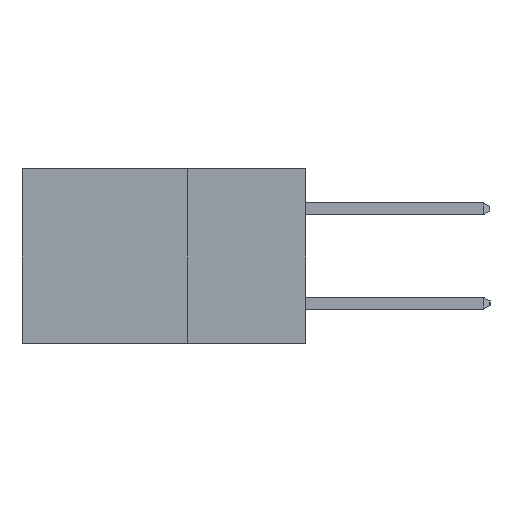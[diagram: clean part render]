
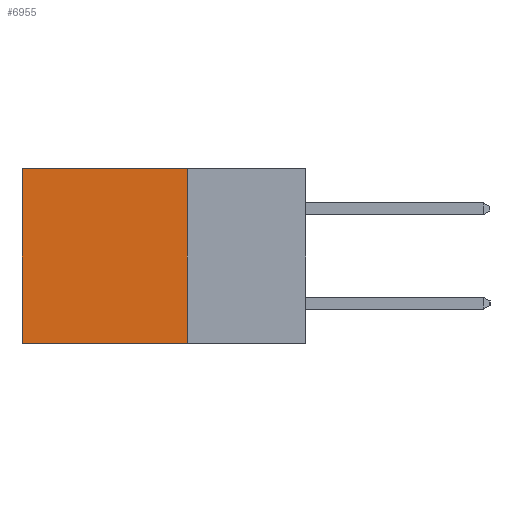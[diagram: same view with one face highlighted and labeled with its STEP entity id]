
A CAD part, left-side view. The second image highlights one B-rep face of the part: STEP entity #6955.
In plain terms, the highlighted planar face has unit normal (-1, 0, 0).
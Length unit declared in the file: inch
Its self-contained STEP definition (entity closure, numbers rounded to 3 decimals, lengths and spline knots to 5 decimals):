
#86 = DIRECTION ( 'NONE',  ( 0., 0., -1. ) ) ;
#236 = DIRECTION ( 'NONE',  ( 0., 1., 0. ) ) ;
#272 = VECTOR ( 'NONE', #14506, 39.37008 ) ;
#843 = EDGE_CURVE ( 'NONE', #16257, #17080, #6444, .T. ) ;
#2298 = ORIENTED_EDGE ( 'NONE', *, *, #8018, .T. ) ;
#2375 = ORIENTED_EDGE ( 'NONE', *, *, #7403, .F. ) ;
#3599 = ORIENTED_EDGE ( 'NONE', *, *, #843, .F. ) ;
#4189 = AXIS2_PLACEMENT_3D ( 'NONE', #18038, #9099, #86 ) ;
#5634 = VERTEX_POINT ( 'NONE', #14897 ) ;
#6444 = LINE ( 'NONE', #7843, #17875 ) ;
#6703 = FACE_OUTER_BOUND ( 'NONE', #10856, .T. ) ;
#6955 = ADVANCED_FACE ( 'NONE', ( #6703 ), #13553, .F. ) ;
#7081 = CARTESIAN_POINT ( 'NONE',  ( 0.2615, 0.25, -0.37 ) ) ;
#7403 = EDGE_CURVE ( 'NONE', #17080, #13776, #12292, .T. ) ;
#7843 = CARTESIAN_POINT ( 'NONE',  ( 0.2615, 0.25, -0.37 ) ) ;
#8018 = EDGE_CURVE ( 'NONE', #16257, #5634, #11586, .T. ) ;
#8021 = VECTOR ( 'NONE', #236, 39.37008 ) ;
#8830 = CARTESIAN_POINT ( 'NONE',  ( 0.2615, 0.6, -0.37 ) ) ;
#9099 = DIRECTION ( 'NONE',  ( 1., 0., 0. ) ) ;
#9244 = CARTESIAN_POINT ( 'NONE',  ( 0.2615, 0.25, 0. ) ) ;
#10377 = DIRECTION ( 'NONE',  ( 0., 0., -1. ) ) ;
#10468 = EDGE_CURVE ( 'NONE', #5634, #13776, #11732, .T. ) ;
#10856 = EDGE_LOOP ( 'NONE', ( #12960, #2375, #3599, #2298 ) ) ;
#11269 = VECTOR ( 'NONE', #10377, 39.37008 ) ;
#11586 = LINE ( 'NONE', #9244, #8021 ) ;
#11732 = LINE ( 'NONE', #8830, #11269 ) ;
#12292 = LINE ( 'NONE', #7081, #272 ) ;
#12680 = CARTESIAN_POINT ( 'NONE',  ( 0.2615, 0.6, -0.37 ) ) ;
#12960 = ORIENTED_EDGE ( 'NONE', *, *, #10468, .T. ) ;
#13553 = PLANE ( 'NONE',  #4189 ) ;
#13776 = VERTEX_POINT ( 'NONE', #12680 ) ;
#14189 = CARTESIAN_POINT ( 'NONE',  ( 0.2615, 0.25, 0. ) ) ;
#14506 = DIRECTION ( 'NONE',  ( 0., 1., 0. ) ) ;
#14897 = CARTESIAN_POINT ( 'NONE',  ( 0.2615, 0.6, 0. ) ) ;
#15748 = CARTESIAN_POINT ( 'NONE',  ( 0.2615, 0.25, -0.37 ) ) ;
#16257 = VERTEX_POINT ( 'NONE', #14189 ) ;
#17080 = VERTEX_POINT ( 'NONE', #15748 ) ;
#17875 = VECTOR ( 'NONE', #18409, 39.37008 ) ;
#18038 = CARTESIAN_POINT ( 'NONE',  ( 0.2615, 0.25, -0.37 ) ) ;
#18409 = DIRECTION ( 'NONE',  ( 0., 0., -1. ) ) ;
